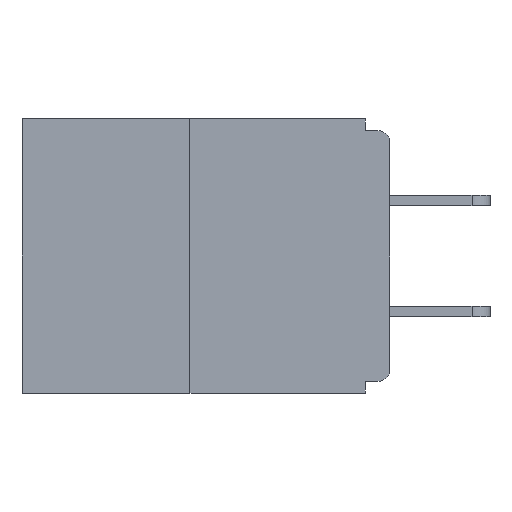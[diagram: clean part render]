
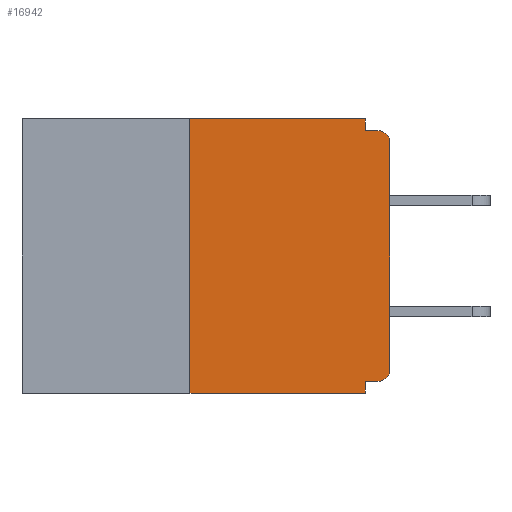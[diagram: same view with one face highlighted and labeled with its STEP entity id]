
A CAD part, left-side view. The second image highlights one B-rep face of the part: STEP entity #16942.
In plain terms, the highlighted planar face has unit normal (-1, 0, 0).
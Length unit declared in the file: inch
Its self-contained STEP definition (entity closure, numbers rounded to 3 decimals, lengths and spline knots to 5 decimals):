
#110 = VERTEX_POINT ( 'NONE', #9840 ) ;
#534 = VERTEX_POINT ( 'NONE', #18480 ) ;
#1334 = CARTESIAN_POINT ( 'NONE',  ( 0., 0.46, 0. ) ) ;
#1707 = EDGE_CURVE ( 'NONE', #21471, #23146, #22686, .T. ) ;
#1820 = VECTOR ( 'NONE', #8180, 39.37008 ) ;
#1827 = VERTEX_POINT ( 'NONE', #23230 ) ;
#1834 = DIRECTION ( 'NONE',  ( 0., 0., -1. ) ) ;
#2054 = CARTESIAN_POINT ( 'NONE',  ( 0., 0.031, 0. ) ) ;
#2073 = ORIENTED_EDGE ( 'NONE', *, *, #4000, .F. ) ;
#2431 = CARTESIAN_POINT ( 'NONE',  ( 0., 0.031, 0. ) ) ;
#3027 = VERTEX_POINT ( 'NONE', #10100 ) ;
#3699 = AXIS2_PLACEMENT_3D ( 'NONE', #25736, #23475, #17559 ) ;
#3981 = EDGE_CURVE ( 'NONE', #534, #23146, #12925, .T. ) ;
#4000 = EDGE_CURVE ( 'NONE', #15351, #1827, #8037, .T. ) ;
#4736 = ORIENTED_EDGE ( 'NONE', *, *, #20971, .T. ) ;
#5594 = CARTESIAN_POINT ( 'NONE',  ( 0., 0., -0.328 ) ) ;
#7727 = ORIENTED_EDGE ( 'NONE', *, *, #22198, .F. ) ;
#7968 = ORIENTED_EDGE ( 'NONE', *, *, #23445, .F. ) ;
#8037 = LINE ( 'NONE', #22812, #1820 ) ;
#8180 = DIRECTION ( 'NONE',  ( 0., -1., 0. ) ) ;
#8509 = CARTESIAN_POINT ( 'NONE',  ( 0., 0.031, -0.343 ) ) ;
#8737 = DIRECTION ( 'NONE',  ( 0., 0., -1. ) ) ;
#9313 = VECTOR ( 'NONE', #14394, 39.37008 ) ;
#9477 = EDGE_CURVE ( 'NONE', #19561, #21471, #11353, .T. ) ;
#9819 = DIRECTION ( 'NONE',  ( 0., 1., 0. ) ) ;
#9840 = CARTESIAN_POINT ( 'NONE',  ( 0., 0., -0.313 ) ) ;
#10100 = CARTESIAN_POINT ( 'NONE',  ( 0., 0.25, 0. ) ) ;
#10366 = VECTOR ( 'NONE', #12955, 39.37008 ) ;
#11353 = LINE ( 'NONE', #5594, #21925 ) ;
#12199 = FACE_OUTER_BOUND ( 'NONE', #19061, .T. ) ;
#12721 = PLANE ( 'NONE',  #23748 ) ;
#12907 = DIRECTION ( 'NONE',  ( 1., 0., 0. ) ) ;
#12923 = ORIENTED_EDGE ( 'NONE', *, *, #17834, .T. ) ;
#12925 = LINE ( 'NONE', #16439, #9313 ) ;
#12955 = DIRECTION ( 'NONE',  ( 0., 0., 1. ) ) ;
#12960 = CIRCLE ( 'NONE', #3699, 0.015 ) ;
#13075 = LINE ( 'NONE', #2431, #23703 ) ;
#13296 = CARTESIAN_POINT ( 'NONE',  ( 0., 0.25, 0. ) ) ;
#13947 = EDGE_CURVE ( 'NONE', #110, #15776, #21249, .T. ) ;
#14394 = DIRECTION ( 'NONE',  ( 0., -1., 0. ) ) ;
#14503 = CARTESIAN_POINT ( 'NONE',  ( 0., 0., -0.03 ) ) ;
#14534 = AXIS2_PLACEMENT_3D ( 'NONE', #22832, #15198, #16364 ) ;
#15198 = DIRECTION ( 'NONE',  ( -1., 0., 0. ) ) ;
#15211 = CARTESIAN_POINT ( 'NONE',  ( 0., 0.031, -0.328 ) ) ;
#15351 = VERTEX_POINT ( 'NONE', #27253 ) ;
#15776 = VERTEX_POINT ( 'NONE', #14503 ) ;
#16364 = DIRECTION ( 'NONE',  ( 0., 0., -1. ) ) ;
#16439 = CARTESIAN_POINT ( 'NONE',  ( 0., 0.46, -0.343 ) ) ;
#16835 = ORIENTED_EDGE ( 'NONE', *, *, #27046, .F. ) ;
#16942 = ADVANCED_FACE ( 'NONE', ( #12199 ), #12721, .F. ) ;
#17559 = DIRECTION ( 'NONE',  ( 0., 0., -1. ) ) ;
#17691 = VERTEX_POINT ( 'NONE', #2054 ) ;
#17834 = EDGE_CURVE ( 'NONE', #19561, #110, #23057, .T. ) ;
#18043 = VECTOR ( 'NONE', #1834, 39.37008 ) ;
#18480 = CARTESIAN_POINT ( 'NONE',  ( 0., 0.25, -0.343 ) ) ;
#18747 = VECTOR ( 'NONE', #26529, 39.37008 ) ;
#19061 = EDGE_LOOP ( 'NONE', ( #16835, #7727, #19436, #26209, #24419, #12923, #26848, #4736, #2073, #7968 ) ) ;
#19177 = CARTESIAN_POINT ( 'NONE',  ( 0., 0., 0. ) ) ;
#19436 = ORIENTED_EDGE ( 'NONE', *, *, #3981, .T. ) ;
#19561 = VERTEX_POINT ( 'NONE', #24153 ) ;
#19728 = LINE ( 'NONE', #1334, #18747 ) ;
#19999 = VECTOR ( 'NONE', #22065, 39.37008 ) ;
#20971 = EDGE_CURVE ( 'NONE', #15776, #1827, #12960, .T. ) ;
#21249 = LINE ( 'NONE', #19177, #10366 ) ;
#21308 = DIRECTION ( 'NONE',  ( 0., 0., -1. ) ) ;
#21467 = CARTESIAN_POINT ( 'NONE',  ( 0., 0.031, -0.343 ) ) ;
#21471 = VERTEX_POINT ( 'NONE', #15211 ) ;
#21925 = VECTOR ( 'NONE', #9819, 39.37008 ) ;
#22065 = DIRECTION ( 'NONE',  ( 0., 0., 1. ) ) ;
#22198 = EDGE_CURVE ( 'NONE', #534, #3027, #25710, .T. ) ;
#22686 = LINE ( 'NONE', #8509, #18043 ) ;
#22812 = CARTESIAN_POINT ( 'NONE',  ( 0., 0., -0.015 ) ) ;
#22832 = CARTESIAN_POINT ( 'NONE',  ( 0., 0.015, -0.313 ) ) ;
#23057 = CIRCLE ( 'NONE', #14534, 0.015 ) ;
#23146 = VERTEX_POINT ( 'NONE', #21467 ) ;
#23230 = CARTESIAN_POINT ( 'NONE',  ( 0., 0.015, -0.015 ) ) ;
#23445 = EDGE_CURVE ( 'NONE', #17691, #15351, #13075, .T. ) ;
#23475 = DIRECTION ( 'NONE',  ( -1., 0., 0. ) ) ;
#23703 = VECTOR ( 'NONE', #8737, 39.37008 ) ;
#23748 = AXIS2_PLACEMENT_3D ( 'NONE', #25640, #12907, #21308 ) ;
#24153 = CARTESIAN_POINT ( 'NONE',  ( 0., 0.015, -0.328 ) ) ;
#24419 = ORIENTED_EDGE ( 'NONE', *, *, #9477, .F. ) ;
#25640 = CARTESIAN_POINT ( 'NONE',  ( 0., 0.46, 0. ) ) ;
#25710 = LINE ( 'NONE', #13296, #19999 ) ;
#25736 = CARTESIAN_POINT ( 'NONE',  ( 0., 0.015, -0.03 ) ) ;
#26209 = ORIENTED_EDGE ( 'NONE', *, *, #1707, .F. ) ;
#26529 = DIRECTION ( 'NONE',  ( 0., -1., 0. ) ) ;
#26848 = ORIENTED_EDGE ( 'NONE', *, *, #13947, .T. ) ;
#27046 = EDGE_CURVE ( 'NONE', #3027, #17691, #19728, .T. ) ;
#27253 = CARTESIAN_POINT ( 'NONE',  ( 0., 0.031, -0.015 ) ) ;
